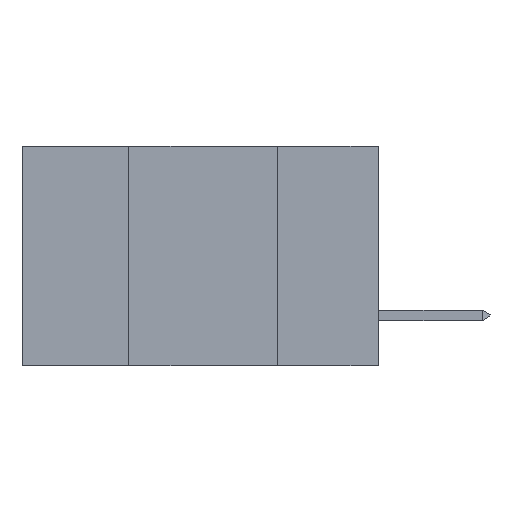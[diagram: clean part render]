
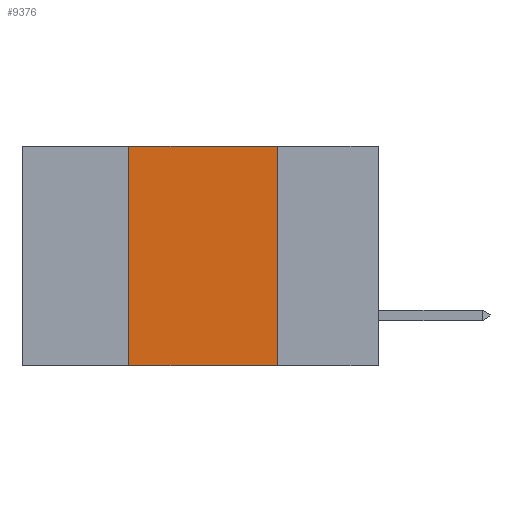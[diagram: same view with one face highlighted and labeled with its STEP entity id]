
A CAD part, left-side view. The second image highlights one B-rep face of the part: STEP entity #9376.
In plain terms, the highlighted planar face has unit normal (-1, 0, 0).
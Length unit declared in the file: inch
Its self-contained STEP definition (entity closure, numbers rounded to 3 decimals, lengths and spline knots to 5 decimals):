
#365 = DIRECTION ( 'NONE',  ( 0., 0., -1. ) ) ;
#604 = CARTESIAN_POINT ( 'NONE',  ( 0., 0.17, -0.37 ) ) ;
#1335 = ORIENTED_EDGE ( 'NONE', *, *, #13776, .F. ) ;
#1433 = VERTEX_POINT ( 'NONE', #1722 ) ;
#1722 = CARTESIAN_POINT ( 'NONE',  ( 0., 0.17, 0. ) ) ;
#3747 = ORIENTED_EDGE ( 'NONE', *, *, #9449, .F. ) ;
#3912 = VECTOR ( 'NONE', #4608, 39.37008 ) ;
#4351 = LINE ( 'NONE', #10251, #16772 ) ;
#4608 = DIRECTION ( 'NONE',  ( 0., -1., 0. ) ) ;
#5431 = CARTESIAN_POINT ( 'NONE',  ( 0., 0.42, -0.37 ) ) ;
#6290 = FACE_OUTER_BOUND ( 'NONE', #15767, .T. ) ;
#7697 = LINE ( 'NONE', #9095, #3912 ) ;
#8126 = AXIS2_PLACEMENT_3D ( 'NONE', #14388, #13201, #365 ) ;
#8252 = VERTEX_POINT ( 'NONE', #9821 ) ;
#9095 = CARTESIAN_POINT ( 'NONE',  ( 0., 0.6, 0. ) ) ;
#9376 = ADVANCED_FACE ( 'NONE', ( #6290 ), #16253, .F. ) ;
#9449 = EDGE_CURVE ( 'NONE', #1433, #18117, #12439, .T. ) ;
#9621 = VERTEX_POINT ( 'NONE', #5431 ) ;
#9821 = CARTESIAN_POINT ( 'NONE',  ( 0., 0.42, 0. ) ) ;
#10251 = CARTESIAN_POINT ( 'NONE',  ( 0., 0.6, -0.37 ) ) ;
#10821 = EDGE_CURVE ( 'NONE', #8252, #1433, #7697, .T. ) ;
#11630 = DIRECTION ( 'NONE',  ( 0., -1., 0. ) ) ;
#12131 = EDGE_CURVE ( 'NONE', #9621, #18117, #4351, .T. ) ;
#12439 = LINE ( 'NONE', #14940, #12567 ) ;
#12567 = VECTOR ( 'NONE', #18106, 39.37008 ) ;
#13201 = DIRECTION ( 'NONE',  ( 1., 0., 0. ) ) ;
#13776 = EDGE_CURVE ( 'NONE', #9621, #8252, #15532, .T. ) ;
#14388 = CARTESIAN_POINT ( 'NONE',  ( 0., 0.6, 0. ) ) ;
#14940 = CARTESIAN_POINT ( 'NONE',  ( 0., 0.17, -0.37 ) ) ;
#14998 = ORIENTED_EDGE ( 'NONE', *, *, #10821, .F. ) ;
#15260 = CARTESIAN_POINT ( 'NONE',  ( 0., 0.42, -0.37 ) ) ;
#15532 = LINE ( 'NONE', #15260, #15613 ) ;
#15613 = VECTOR ( 'NONE', #16570, 39.37008 ) ;
#15767 = EDGE_LOOP ( 'NONE', ( #3747, #14998, #1335, #18275 ) ) ;
#16253 = PLANE ( 'NONE',  #8126 ) ;
#16570 = DIRECTION ( 'NONE',  ( 0., 0., 1. ) ) ;
#16772 = VECTOR ( 'NONE', #11630, 39.37008 ) ;
#18106 = DIRECTION ( 'NONE',  ( 0., 0., -1. ) ) ;
#18117 = VERTEX_POINT ( 'NONE', #604 ) ;
#18275 = ORIENTED_EDGE ( 'NONE', *, *, #12131, .T. ) ;
